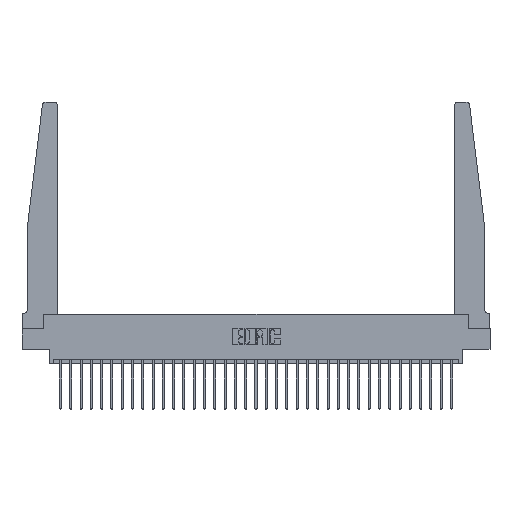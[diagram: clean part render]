
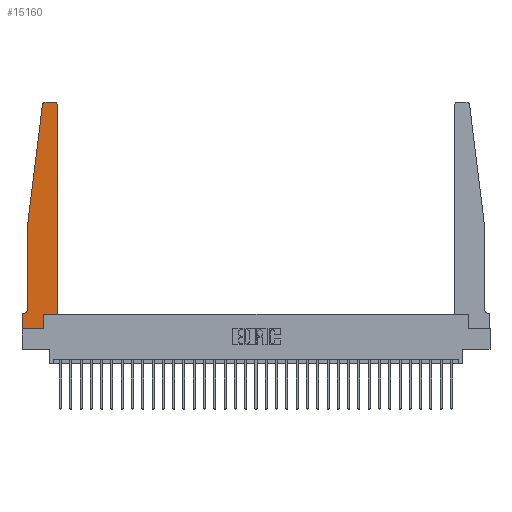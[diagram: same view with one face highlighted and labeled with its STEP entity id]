
A CAD part, top view. The second image highlights one B-rep face of the part: STEP entity #15160.
In plain terms, the highlighted planar face has unit normal (0, 0, 1).
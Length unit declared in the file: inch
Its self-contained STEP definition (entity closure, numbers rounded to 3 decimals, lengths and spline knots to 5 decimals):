
#399 = CIRCLE ( 'NONE', #24765, 0.05 ) ;
#558 = VECTOR ( 'NONE', #26396, 39.37008 ) ;
#1319 = LINE ( 'NONE', #7353, #558 ) ;
#1592 = LINE ( 'NONE', #4235, #19081 ) ;
#1898 = EDGE_LOOP ( 'NONE', ( #2835, #8269, #12693, #16601, #27380, #15058, #9115, #19360, #10363, #14557, #30194, #8811 ) ) ;
#2575 = EDGE_CURVE ( 'NONE', #12056, #19836, #16165, .T. ) ;
#2835 = ORIENTED_EDGE ( 'NONE', *, *, #28898, .T. ) ;
#2847 = DIRECTION ( 'NONE',  ( -1., 0., 0. ) ) ;
#3193 = VERTEX_POINT ( 'NONE', #10308 ) ;
#3366 = CARTESIAN_POINT ( 'NONE',  ( 0.065, 1.25, 0.37 ) ) ;
#3635 = EDGE_CURVE ( 'NONE', #16990, #12056, #25395, .T. ) ;
#4107 = CARTESIAN_POINT ( 'NONE',  ( 0.2605, 0., 0.37 ) ) ;
#4235 = CARTESIAN_POINT ( 'NONE',  ( 0.425, 0.18, 0.37 ) ) ;
#4690 = VECTOR ( 'NONE', #25731, 39.37008 ) ;
#5346 = CARTESIAN_POINT ( 'NONE',  ( 0., 0., 0.37 ) ) ;
#5701 = CARTESIAN_POINT ( 'NONE',  ( 0., 0.1875, 0.37 ) ) ;
#5733 = CIRCLE ( 'NONE', #17033, 0.03 ) ;
#5914 = DIRECTION ( 'NONE',  ( -0.122, -0.992, 0. ) ) ;
#6402 = VERTEX_POINT ( 'NONE', #12886 ) ;
#6636 = DIRECTION ( 'NONE',  ( 0., 1., 0. ) ) ;
#6832 = CARTESIAN_POINT ( 'NONE',  ( 0.24675, 2.72367, 0.37 ) ) ;
#6879 = CARTESIAN_POINT ( 'NONE',  ( 0., 0.1875, 0.37 ) ) ;
#6908 = AXIS2_PLACEMENT_3D ( 'NONE', #6879, #25919, #11668 ) ;
#7134 = DIRECTION ( 'NONE',  ( -1., 0., 0. ) ) ;
#7185 = DIRECTION ( 'NONE',  ( 0., 0., -1. ) ) ;
#7237 = CARTESIAN_POINT ( 'NONE',  ( 0.065, 0.2375, 0.37 ) ) ;
#7353 = CARTESIAN_POINT ( 'NONE',  ( 0.2605, 0.18, 0.37 ) ) ;
#7888 = EDGE_CURVE ( 'NONE', #12422, #12320, #11034, .T. ) ;
#8269 = ORIENTED_EDGE ( 'NONE', *, *, #24436, .T. ) ;
#8730 = EDGE_CURVE ( 'NONE', #19836, #12422, #1319, .T. ) ;
#8811 = ORIENTED_EDGE ( 'NONE', *, *, #13955, .T. ) ;
#9115 = ORIENTED_EDGE ( 'NONE', *, *, #3635, .T. ) ;
#9776 = CARTESIAN_POINT ( 'NONE',  ( 0., 0., 0.37 ) ) ;
#10308 = CARTESIAN_POINT ( 'NONE',  ( 0.425, 2.72, 0.37 ) ) ;
#10363 = ORIENTED_EDGE ( 'NONE', *, *, #8730, .T. ) ;
#10781 = VERTEX_POINT ( 'NONE', #3366 ) ;
#11034 = LINE ( 'NONE', #29974, #4690 ) ;
#11134 = EDGE_CURVE ( 'NONE', #30706, #16526, #399, .T. ) ;
#11217 = CARTESIAN_POINT ( 'NONE',  ( 0.27653, 2.72, 0.37 ) ) ;
#11668 = DIRECTION ( 'NONE',  ( 1., 0., 0. ) ) ;
#12056 = VERTEX_POINT ( 'NONE', #24741 ) ;
#12320 = VERTEX_POINT ( 'NONE', #18494 ) ;
#12422 = VERTEX_POINT ( 'NONE', #21087 ) ;
#12693 = ORIENTED_EDGE ( 'NONE', *, *, #15512, .T. ) ;
#12755 = LINE ( 'NONE', #17111, #19087 ) ;
#12886 = CARTESIAN_POINT ( 'NONE',  ( 0.395, 2.75, 0.37 ) ) ;
#13617 = DIRECTION ( 'NONE',  ( 1., 0., 0. ) ) ;
#13635 = DIRECTION ( 'NONE',  ( 0., -1., 0. ) ) ;
#13805 = DIRECTION ( 'NONE',  ( 0., 0., 1. ) ) ;
#13948 = EDGE_CURVE ( 'NONE', #12320, #3193, #1592, .T. ) ;
#13955 = EDGE_CURVE ( 'NONE', #3193, #6402, #25409, .T. ) ;
#14021 = VERTEX_POINT ( 'NONE', #6832 ) ;
#14557 = ORIENTED_EDGE ( 'NONE', *, *, #7888, .T. ) ;
#14683 = EDGE_CURVE ( 'NONE', #16526, #16990, #12755, .T. ) ;
#15058 = ORIENTED_EDGE ( 'NONE', *, *, #14683, .T. ) ;
#15160 = ADVANCED_FACE ( 'NONE', ( #19056 ), #23530, .T. ) ;
#15512 = EDGE_CURVE ( 'NONE', #14021, #10781, #22761, .T. ) ;
#15672 = VECTOR ( 'NONE', #5914, 39.37008 ) ;
#16165 = LINE ( 'NONE', #5346, #28050 ) ;
#16526 = VERTEX_POINT ( 'NONE', #28087 ) ;
#16601 = ORIENTED_EDGE ( 'NONE', *, *, #26305, .T. ) ;
#16990 = VERTEX_POINT ( 'NONE', #5701 ) ;
#17033 = AXIS2_PLACEMENT_3D ( 'NONE', #11217, #27852, #13617 ) ;
#17111 = CARTESIAN_POINT ( 'NONE',  ( 0.065, 0.1875, 0.37 ) ) ;
#17800 = CARTESIAN_POINT ( 'NONE',  ( 0.065, 1.25, 0.37 ) ) ;
#18494 = CARTESIAN_POINT ( 'NONE',  ( 0.425, 0.18, 0.37 ) ) ;
#19056 = FACE_OUTER_BOUND ( 'NONE', #1898, .T. ) ;
#19066 = VECTOR ( 'NONE', #24037, 39.37008 ) ;
#19081 = VECTOR ( 'NONE', #6636, 39.37008 ) ;
#19087 = VECTOR ( 'NONE', #2847, 39.37008 ) ;
#19360 = ORIENTED_EDGE ( 'NONE', *, *, #2575, .T. ) ;
#19620 = DIRECTION ( 'NONE',  ( 1., 0., 0. ) ) ;
#19836 = VERTEX_POINT ( 'NONE', #4107 ) ;
#21087 = CARTESIAN_POINT ( 'NONE',  ( 0.2605, 0.18, 0.37 ) ) ;
#21215 = VECTOR ( 'NONE', #13635, 39.37008 ) ;
#21450 = CARTESIAN_POINT ( 'NONE',  ( 0.015, 0.2375, 0.37 ) ) ;
#21957 = LINE ( 'NONE', #25513, #21215 ) ;
#22761 = LINE ( 'NONE', #17800, #15672 ) ;
#23530 = PLANE ( 'NONE',  #6908 ) ;
#23790 = CARTESIAN_POINT ( 'NONE',  ( 0.25, 2.75, 0.37 ) ) ;
#23844 = DIRECTION ( 'NONE',  ( -1., 0., 0. ) ) ;
#24037 = DIRECTION ( 'NONE',  ( 0., -1., 0. ) ) ;
#24436 = EDGE_CURVE ( 'NONE', #26196, #14021, #5733, .T. ) ;
#24741 = CARTESIAN_POINT ( 'NONE',  ( 0., 0., 0.37 ) ) ;
#24765 = AXIS2_PLACEMENT_3D ( 'NONE', #21450, #7185, #23844 ) ;
#25395 = LINE ( 'NONE', #9776, #19066 ) ;
#25409 = CIRCLE ( 'NONE', #26817, 0.03 ) ;
#25513 = CARTESIAN_POINT ( 'NONE',  ( 0.065, 1.25, 0.37 ) ) ;
#25731 = DIRECTION ( 'NONE',  ( 1., 0., 0. ) ) ;
#25919 = DIRECTION ( 'NONE',  ( 0., 0., 1. ) ) ;
#26196 = VERTEX_POINT ( 'NONE', #27471 ) ;
#26260 = VECTOR ( 'NONE', #7134, 39.37008 ) ;
#26305 = EDGE_CURVE ( 'NONE', #10781, #30706, #21957, .T. ) ;
#26396 = DIRECTION ( 'NONE',  ( 0., 1., 0. ) ) ;
#26817 = AXIS2_PLACEMENT_3D ( 'NONE', #28047, #13805, #30427 ) ;
#26990 = LINE ( 'NONE', #23790, #26260 ) ;
#27380 = ORIENTED_EDGE ( 'NONE', *, *, #11134, .T. ) ;
#27471 = CARTESIAN_POINT ( 'NONE',  ( 0.27653, 2.75, 0.37 ) ) ;
#27852 = DIRECTION ( 'NONE',  ( 0., 0., 1. ) ) ;
#28047 = CARTESIAN_POINT ( 'NONE',  ( 0.395, 2.72, 0.37 ) ) ;
#28050 = VECTOR ( 'NONE', #19620, 39.37008 ) ;
#28087 = CARTESIAN_POINT ( 'NONE',  ( 0.015, 0.1875, 0.37 ) ) ;
#28898 = EDGE_CURVE ( 'NONE', #6402, #26196, #26990, .T. ) ;
#29974 = CARTESIAN_POINT ( 'NONE',  ( 0.425, 0.18, 0.37 ) ) ;
#30194 = ORIENTED_EDGE ( 'NONE', *, *, #13948, .T. ) ;
#30427 = DIRECTION ( 'NONE',  ( 1., 0., 0. ) ) ;
#30706 = VERTEX_POINT ( 'NONE', #7237 ) ;
